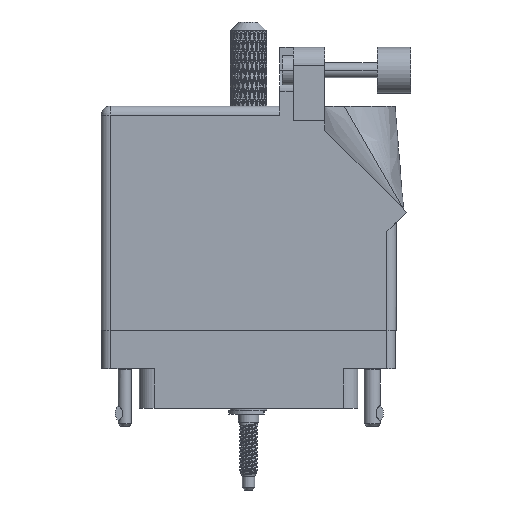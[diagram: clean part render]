
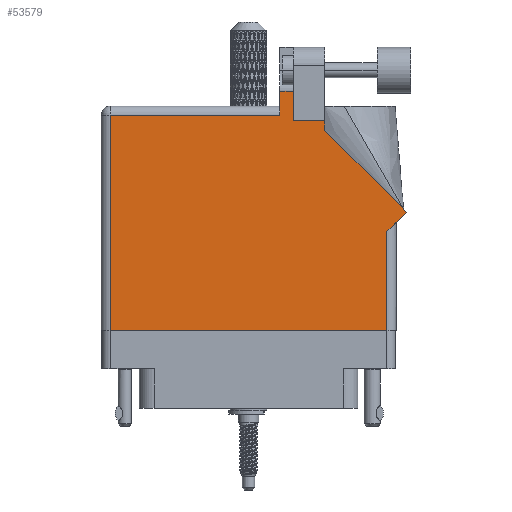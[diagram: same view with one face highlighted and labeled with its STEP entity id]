
A CAD part, front view. The second image highlights one B-rep face of the part: STEP entity #53579.
In plain terms, the highlighted face is planar.
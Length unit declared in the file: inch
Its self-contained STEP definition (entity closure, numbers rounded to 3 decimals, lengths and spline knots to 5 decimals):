
#135 = CARTESIAN_POINT ( 'NONE',  ( 1.948, 0.675, 0. ) ) ;
#771 = DIRECTION ( 'NONE',  ( -1., 0., 0. ) ) ;
#824 = ORIENTED_EDGE ( 'NONE', *, *, #75484, .T. ) ;
#3430 = CARTESIAN_POINT ( 'NONE',  ( 1.948, 0., 0. ) ) ;
#4069 = LINE ( 'NONE', #70497, #39758 ) ;
#4491 = LINE ( 'NONE', #49471, #11289 ) ;
#4785 = CARTESIAN_POINT ( 'NONE',  ( 1.311, 1.43, 0. ) ) ;
#5507 = DIRECTION ( 'NONE',  ( 0., 0., -1. ) ) ;
#5714 = DIRECTION ( 'NONE',  ( -1., 0., 0. ) ) ;
#6358 = CARTESIAN_POINT ( 'NONE',  ( 0.062, 0., 0. ) ) ;
#8187 = CARTESIAN_POINT ( 'NONE',  ( 1.311, 1.6315, 0. ) ) ;
#9054 = VECTOR ( 'NONE', #95845, 39.37008 ) ;
#10806 = DIRECTION ( 'NONE',  ( 1., 0., 0. ) ) ;
#10881 = VERTEX_POINT ( 'NONE', #112028 ) ;
#11289 = VECTOR ( 'NONE', #5714, 39.37008 ) ;
#12470 = CARTESIAN_POINT ( 'NONE',  ( 1.311, 1.43, 0. ) ) ;
#21867 = ORIENTED_EDGE ( 'NONE', *, *, #90730, .T. ) ;
#25298 = ORIENTED_EDGE ( 'NONE', *, *, #72900, .T. ) ;
#26375 = ORIENTED_EDGE ( 'NONE', *, *, #63817, .T. ) ;
#27974 = EDGE_CURVE ( 'NONE', #62465, #89487, #51478, .T. ) ;
#28067 = VECTOR ( 'NONE', #49312, 39.37008 ) ;
#28192 = LINE ( 'NONE', #4785, #111009 ) ;
#28262 = ORIENTED_EDGE ( 'NONE', *, *, #111819, .T. ) ;
#29444 = AXIS2_PLACEMENT_3D ( 'NONE', #84784, #5507, #48469 ) ;
#30128 = EDGE_CURVE ( 'NONE', #49878, #67473, #70503, .T. ) ;
#36712 = CARTESIAN_POINT ( 'NONE',  ( 1.64177, 1.6315, 0. ) ) ;
#37013 = DIRECTION ( 'NONE',  ( 0., 1., 0. ) ) ;
#38343 = VERTEX_POINT ( 'NONE', #55111 ) ;
#38427 = VERTEX_POINT ( 'NONE', #12470 ) ;
#39758 = VECTOR ( 'NONE', #771, 39.37008 ) ;
#40428 = ORIENTED_EDGE ( 'NONE', *, *, #105674, .T. ) ;
#40429 = CARTESIAN_POINT ( 'NONE',  ( 1.524, 1.36442, 0. ) ) ;
#41073 = CARTESIAN_POINT ( 'NONE',  ( 1.948, 0.737, 0. ) ) ;
#43059 = DIRECTION ( 'NONE',  ( -0.707, 0.707, 0. ) ) ;
#45120 = DIRECTION ( 'NONE',  ( -1., 0., 0. ) ) ;
#45803 = LINE ( 'NONE', #75223, #59733 ) ;
#48469 = DIRECTION ( 'NONE',  ( -1., 0., 0. ) ) ;
#48847 = EDGE_CURVE ( 'NONE', #105297, #113489, #59967, .T. ) ;
#49312 = DIRECTION ( 'NONE',  ( 0., 1., 0. ) ) ;
#49471 = CARTESIAN_POINT ( 'NONE',  ( 0., 1.468, 0. ) ) ;
#49878 = VERTEX_POINT ( 'NONE', #8187 ) ;
#51478 = LINE ( 'NONE', #60599, #105354 ) ;
#52420 = VECTOR ( 'NONE', #57316, 39.37008 ) ;
#53579 = ADVANCED_FACE ( 'NONE', ( #113431 ), #101397, .F. ) ;
#55111 = CARTESIAN_POINT ( 'NONE',  ( 1.524, 1.36442, 0. ) ) ;
#55156 = LINE ( 'NONE', #41073, #52420 ) ;
#56240 = LINE ( 'NONE', #64630, #78518 ) ;
#57316 = DIRECTION ( 'NONE',  ( 0., 1., 0. ) ) ;
#59733 = VECTOR ( 'NONE', #43059, 39.37008 ) ;
#59788 = ORIENTED_EDGE ( 'NONE', *, *, #27974, .T. ) ;
#59967 = LINE ( 'NONE', #96576, #9054 ) ;
#60599 = CARTESIAN_POINT ( 'NONE',  ( 0.062, 0., 0. ) ) ;
#62465 = VERTEX_POINT ( 'NONE', #75604 ) ;
#63817 = EDGE_CURVE ( 'NONE', #113489, #38343, #45803, .T. ) ;
#64630 = CARTESIAN_POINT ( 'NONE',  ( 0., 0., 0. ) ) ;
#67473 = VERTEX_POINT ( 'NONE', #67939 ) ;
#67939 = CARTESIAN_POINT ( 'NONE',  ( 1.217, 1.6315, 0. ) ) ;
#68589 = DIRECTION ( 'NONE',  ( 0., -1., 0. ) ) ;
#70497 = CARTESIAN_POINT ( 'NONE',  ( 1.524, 1.43, 0. ) ) ;
#70503 = LINE ( 'NONE', #36712, #91153 ) ;
#71290 = CARTESIAN_POINT ( 'NONE',  ( 1.524, 1.43, 0. ) ) ;
#72900 = EDGE_CURVE ( 'NONE', #38427, #49878, #28192, .T. ) ;
#73039 = EDGE_CURVE ( 'NONE', #38343, #102479, #83238, .T. ) ;
#75223 = CARTESIAN_POINT ( 'NONE',  ( 2.08071, 0.80771, 0. ) ) ;
#75484 = EDGE_CURVE ( 'NONE', #10881, #62465, #4491, .T. ) ;
#75604 = CARTESIAN_POINT ( 'NONE',  ( 0.062, 1.468, 0. ) ) ;
#78518 = VECTOR ( 'NONE', #10806, 39.37008 ) ;
#80683 = ORIENTED_EDGE ( 'NONE', *, *, #48847, .T. ) ;
#83238 = LINE ( 'NONE', #40429, #28067 ) ;
#84784 = CARTESIAN_POINT ( 'NONE',  ( 0., 1.53, 0. ) ) ;
#87012 = CARTESIAN_POINT ( 'NONE',  ( 2.08071, 0.80771, 0. ) ) ;
#89487 = VERTEX_POINT ( 'NONE', #6358 ) ;
#90730 = EDGE_CURVE ( 'NONE', #102479, #38427, #4069, .T. ) ;
#91153 = VECTOR ( 'NONE', #45120, 39.37008 ) ;
#93190 = EDGE_LOOP ( 'NONE', ( #25298, #101096, #28262, #824, #59788, #40428, #97242, #80683, #26375, #113664, #21867 ) ) ;
#94374 = LINE ( 'NONE', #103696, #101191 ) ;
#95010 = EDGE_CURVE ( 'NONE', #107496, #105297, #55156, .T. ) ;
#95845 = DIRECTION ( 'NONE',  ( 0.707, 0.707, 0. ) ) ;
#96576 = CARTESIAN_POINT ( 'NONE',  ( 2.01, 0.737, 0. ) ) ;
#97233 = DIRECTION ( 'NONE',  ( 0., -1., 0. ) ) ;
#97242 = ORIENTED_EDGE ( 'NONE', *, *, #95010, .T. ) ;
#101096 = ORIENTED_EDGE ( 'NONE', *, *, #30128, .T. ) ;
#101191 = VECTOR ( 'NONE', #68589, 39.37008 ) ;
#101397 = PLANE ( 'NONE',  #29444 ) ;
#102479 = VERTEX_POINT ( 'NONE', #71290 ) ;
#103696 = CARTESIAN_POINT ( 'NONE',  ( 1.217, 1.53, 0. ) ) ;
#105297 = VERTEX_POINT ( 'NONE', #135 ) ;
#105354 = VECTOR ( 'NONE', #97233, 39.37008 ) ;
#105674 = EDGE_CURVE ( 'NONE', #89487, #107496, #56240, .T. ) ;
#107496 = VERTEX_POINT ( 'NONE', #3430 ) ;
#111009 = VECTOR ( 'NONE', #37013, 39.37008 ) ;
#111819 = EDGE_CURVE ( 'NONE', #67473, #10881, #94374, .T. ) ;
#112028 = CARTESIAN_POINT ( 'NONE',  ( 1.217, 1.468, 0. ) ) ;
#113431 = FACE_OUTER_BOUND ( 'NONE', #93190, .T. ) ;
#113489 = VERTEX_POINT ( 'NONE', #87012 ) ;
#113664 = ORIENTED_EDGE ( 'NONE', *, *, #73039, .T. ) ;
